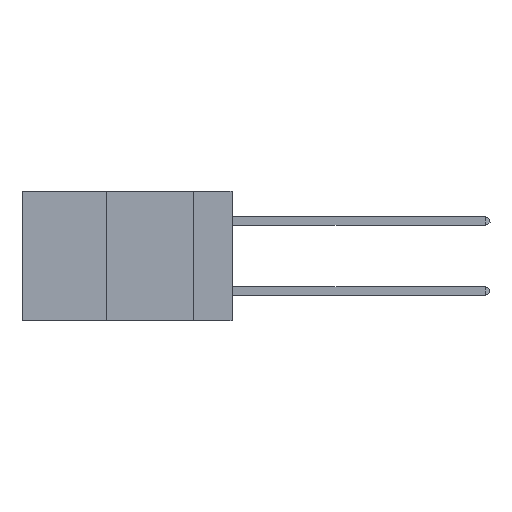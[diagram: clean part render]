
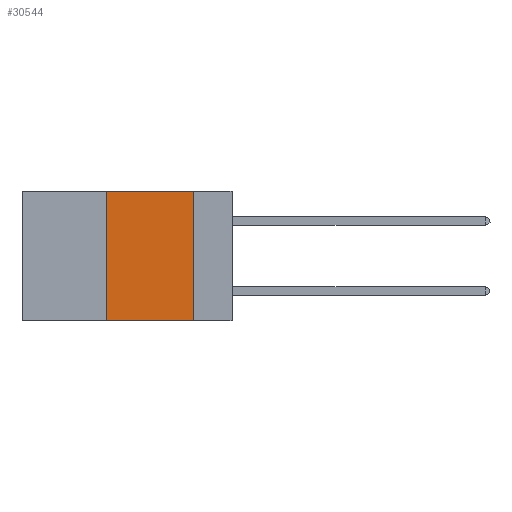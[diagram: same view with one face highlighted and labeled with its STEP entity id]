
A CAD part, left-side view. The second image highlights one B-rep face of the part: STEP entity #30544.
In plain terms, the highlighted planar face has unit normal (-1, 0, 0).
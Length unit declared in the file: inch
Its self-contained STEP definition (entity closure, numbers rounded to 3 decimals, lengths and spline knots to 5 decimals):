
#413 = CARTESIAN_POINT ( 'NONE',  ( 0., 0.36, 0. ) ) ;
#2436 = AXIS2_PLACEMENT_3D ( 'NONE', #29085, #8392, #32198 ) ;
#4210 = CARTESIAN_POINT ( 'NONE',  ( 0., 0.36, -0.37 ) ) ;
#4590 = VERTEX_POINT ( 'NONE', #10454 ) ;
#5127 = CARTESIAN_POINT ( 'NONE',  ( 0., 0.11, 0. ) ) ;
#6428 = LINE ( 'NONE', #12481, #12117 ) ;
#6621 = ORIENTED_EDGE ( 'NONE', *, *, #15481, .T. ) ;
#8337 = LINE ( 'NONE', #38358, #14576 ) ;
#8392 = DIRECTION ( 'NONE',  ( 1., 0., 0. ) ) ;
#8769 = PLANE ( 'NONE',  #2436 ) ;
#10454 = CARTESIAN_POINT ( 'NONE',  ( 0., 0.11, -0.37 ) ) ;
#10985 = EDGE_CURVE ( 'NONE', #35303, #4590, #32272, .T. ) ;
#11583 = DIRECTION ( 'NONE',  ( 0., 0., -1. ) ) ;
#11834 = DIRECTION ( 'NONE',  ( 0., -1., 0. ) ) ;
#12117 = VECTOR ( 'NONE', #15635, 39.37008 ) ;
#12481 = CARTESIAN_POINT ( 'NONE',  ( 0., 0.36, 0. ) ) ;
#14046 = FACE_OUTER_BOUND ( 'NONE', #24060, .T. ) ;
#14576 = VECTOR ( 'NONE', #11834, 39.37008 ) ;
#15002 = EDGE_CURVE ( 'NONE', #30281, #35303, #8337, .T. ) ;
#15481 = EDGE_CURVE ( 'NONE', #23318, #4590, #20792, .T. ) ;
#15635 = DIRECTION ( 'NONE',  ( 0., 0., 1. ) ) ;
#20029 = CARTESIAN_POINT ( 'NONE',  ( 0., 0.11, 0. ) ) ;
#20229 = VECTOR ( 'NONE', #32647, 39.37008 ) ;
#20792 = LINE ( 'NONE', #23901, #20229 ) ;
#22603 = VECTOR ( 'NONE', #11583, 39.37008 ) ;
#23318 = VERTEX_POINT ( 'NONE', #4210 ) ;
#23901 = CARTESIAN_POINT ( 'NONE',  ( 0., 0.6, -0.37 ) ) ;
#24060 = EDGE_LOOP ( 'NONE', ( #34543, #34661, #32058, #6621 ) ) ;
#29085 = CARTESIAN_POINT ( 'NONE',  ( 0., 0.6, 0. ) ) ;
#30281 = VERTEX_POINT ( 'NONE', #413 ) ;
#30544 = ADVANCED_FACE ( 'NONE', ( #14046 ), #8769, .F. ) ;
#32058 = ORIENTED_EDGE ( 'NONE', *, *, #35964, .F. ) ;
#32198 = DIRECTION ( 'NONE',  ( 0., 0., -1. ) ) ;
#32272 = LINE ( 'NONE', #20029, #22603 ) ;
#32647 = DIRECTION ( 'NONE',  ( 0., -1., 0. ) ) ;
#34543 = ORIENTED_EDGE ( 'NONE', *, *, #10985, .F. ) ;
#34661 = ORIENTED_EDGE ( 'NONE', *, *, #15002, .F. ) ;
#35303 = VERTEX_POINT ( 'NONE', #5127 ) ;
#35964 = EDGE_CURVE ( 'NONE', #23318, #30281, #6428, .T. ) ;
#38358 = CARTESIAN_POINT ( 'NONE',  ( 0., 0.6, 0. ) ) ;
